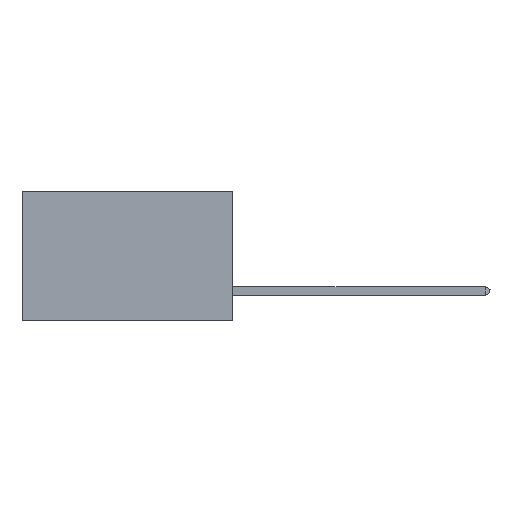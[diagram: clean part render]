
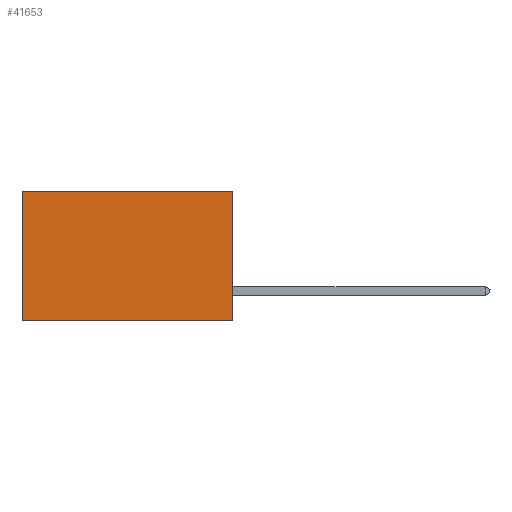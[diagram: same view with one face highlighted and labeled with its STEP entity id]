
A CAD part, left-side view. The second image highlights one B-rep face of the part: STEP entity #41653.
In plain terms, the highlighted planar face has unit normal (-1, 0, 0).
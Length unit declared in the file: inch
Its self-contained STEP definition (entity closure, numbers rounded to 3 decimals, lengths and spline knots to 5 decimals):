
#718 = CARTESIAN_POINT ( 'NONE',  ( 0.2875, 0.6, 0. ) ) ;
#1934 = VECTOR ( 'NONE', #37665, 39.37008 ) ;
#2024 = VECTOR ( 'NONE', #38290, 39.37008 ) ;
#3560 = CARTESIAN_POINT ( 'NONE',  ( 0.2875, 0., 0. ) ) ;
#3618 = CARTESIAN_POINT ( 'NONE',  ( 0.2875, 0., 0. ) ) ;
#7039 = DIRECTION ( 'NONE',  ( 0., 1., 0. ) ) ;
#7111 = VERTEX_POINT ( 'NONE', #3618 ) ;
#7241 = VERTEX_POINT ( 'NONE', #21473 ) ;
#8181 = LINE ( 'NONE', #30627, #36033 ) ;
#9501 = CARTESIAN_POINT ( 'NONE',  ( 0.2875, 0., -0.37 ) ) ;
#10180 = VECTOR ( 'NONE', #26629, 39.37008 ) ;
#10964 = LINE ( 'NONE', #22320, #1934 ) ;
#12223 = FACE_OUTER_BOUND ( 'NONE', #31872, .T. ) ;
#16543 = EDGE_CURVE ( 'NONE', #29164, #26292, #10964, .T. ) ;
#17767 = CARTESIAN_POINT ( 'NONE',  ( 0.2875, 0.6, -0.37 ) ) ;
#18872 = AXIS2_PLACEMENT_3D ( 'NONE', #3560, #20491, #37771 ) ;
#20491 = DIRECTION ( 'NONE',  ( 1., 0., 0. ) ) ;
#21372 = EDGE_CURVE ( 'NONE', #7111, #29164, #8181, .T. ) ;
#21473 = CARTESIAN_POINT ( 'NONE',  ( 0.2875, 0., -0.37 ) ) ;
#22320 = CARTESIAN_POINT ( 'NONE',  ( 0.2875, 0.6, 0. ) ) ;
#22933 = LINE ( 'NONE', #24595, #2024 ) ;
#24595 = CARTESIAN_POINT ( 'NONE',  ( 0.2875, 0., 0. ) ) ;
#26292 = VERTEX_POINT ( 'NONE', #17767 ) ;
#26629 = DIRECTION ( 'NONE',  ( 0., 1., 0. ) ) ;
#28039 = ORIENTED_EDGE ( 'NONE', *, *, #33462, .F. ) ;
#29164 = VERTEX_POINT ( 'NONE', #718 ) ;
#30627 = CARTESIAN_POINT ( 'NONE',  ( 0.2875, 0., 0. ) ) ;
#31872 = EDGE_LOOP ( 'NONE', ( #39192, #37555, #28039, #40475 ) ) ;
#33462 = EDGE_CURVE ( 'NONE', #7111, #7241, #22933, .T. ) ;
#36033 = VECTOR ( 'NONE', #7039, 39.37008 ) ;
#37555 = ORIENTED_EDGE ( 'NONE', *, *, #39697, .F. ) ;
#37665 = DIRECTION ( 'NONE',  ( 0., 0., -1. ) ) ;
#37771 = DIRECTION ( 'NONE',  ( 0., 0., -1. ) ) ;
#38290 = DIRECTION ( 'NONE',  ( 0., 0., -1. ) ) ;
#39192 = ORIENTED_EDGE ( 'NONE', *, *, #16543, .T. ) ;
#39697 = EDGE_CURVE ( 'NONE', #7241, #26292, #41122, .T. ) ;
#40475 = ORIENTED_EDGE ( 'NONE', *, *, #21372, .T. ) ;
#40867 = PLANE ( 'NONE',  #18872 ) ;
#41122 = LINE ( 'NONE', #9501, #10180 ) ;
#41653 = ADVANCED_FACE ( 'NONE', ( #12223 ), #40867, .F. ) ;
